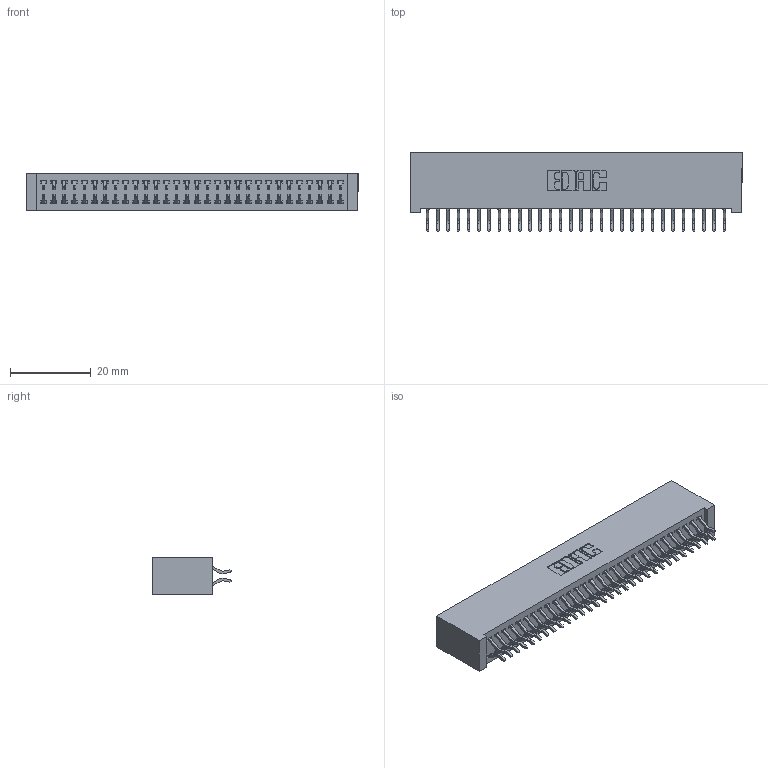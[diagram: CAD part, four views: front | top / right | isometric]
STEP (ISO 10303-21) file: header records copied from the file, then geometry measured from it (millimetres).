
FILE_DESCRIPTION (( 'STEP AP203' ), '1' );
FILE_NAME ('342-060-556-201.STEP', '2018-08-13T06:18:46', ( '' ), ( '' ), 'SwSTEP 2.0', 'SolidWorks 2016', '' );
FILE_SCHEMA (( 'CONFIG_CONTROL_DESIGN' ));
Length unit declared in the file: inch
Products named in the file (3): 342-060-556-201; 342 Part_Lugless; 345-292-001_556 Tail
Assembly tree (61 placements, depth 2):
  342-060-556-201
    342 Part_Lugless
    345-292-001_556 Tail  x60
Bounding box: 82.45 x 19.58 x 9.4 mm (x, y, z)
Volume: 7789.2 mm3; surface area: 12771.2 mm2
Topology: 61 solids, 61 shells, 3582 faces, 10655 edges, 7022 vertices
Faces by surface type: plane 2462, cylinder 1120
Entity records: 20663 total; most frequent: CARTESIAN_POINT 3450, ORIENTED_EDGE 3374, DIRECTION 2951, EDGE_CURVE 1687, VECTOR 1559, LINE 1559, VERTEX_POINT 1122, AXIS2_PLACEMENT_3D 696
